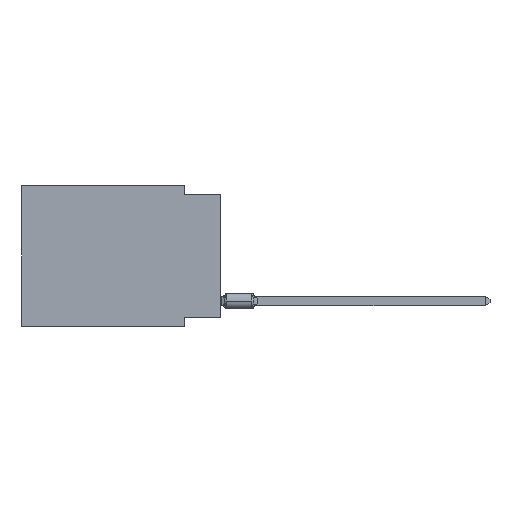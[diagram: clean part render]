
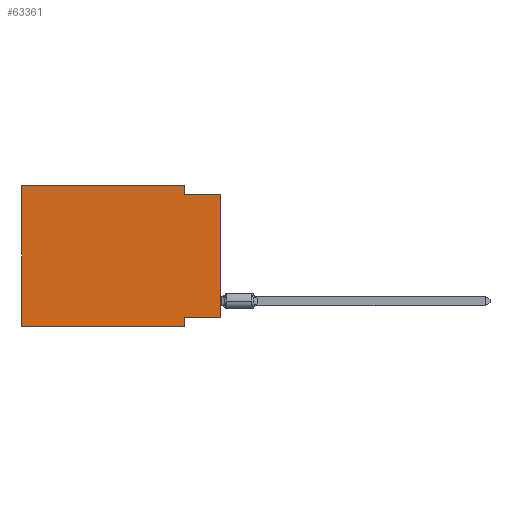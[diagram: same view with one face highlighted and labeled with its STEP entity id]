
A CAD part, left-side view. The second image highlights one B-rep face of the part: STEP entity #63361.
In plain terms, the highlighted planar face has unit normal (-1, 0, 0).
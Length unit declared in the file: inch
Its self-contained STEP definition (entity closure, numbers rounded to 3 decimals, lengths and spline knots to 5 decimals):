
#526 = VECTOR ( 'NONE', #19034, 39.37008 ) ;
#816 = ORIENTED_EDGE ( 'NONE', *, *, #60387, .F. ) ;
#2575 = VERTEX_POINT ( 'NONE', #33905 ) ;
#2750 = VECTOR ( 'NONE', #73653, 39.37008 ) ;
#6491 = CARTESIAN_POINT ( 'NONE',  ( 0., 0.55, 0. ) ) ;
#8063 = EDGE_LOOP ( 'NONE', ( #31172, #16062, #46462, #55585, #9830, #26280, #29709, #816 ) ) ;
#8276 = VERTEX_POINT ( 'NONE', #61489 ) ;
#9830 = ORIENTED_EDGE ( 'NONE', *, *, #71183, .F. ) ;
#11281 = VECTOR ( 'NONE', #72518, 39.37008 ) ;
#12258 = LINE ( 'NONE', #13443, #526 ) ;
#13443 = CARTESIAN_POINT ( 'NONE',  ( 0., 0., 0. ) ) ;
#13620 = LINE ( 'NONE', #6491, #14271 ) ;
#13985 = CARTESIAN_POINT ( 'NONE',  ( 0., 0.1, 0. ) ) ;
#14271 = VECTOR ( 'NONE', #56157, 39.37008 ) ;
#16062 = ORIENTED_EDGE ( 'NONE', *, *, #34835, .F. ) ;
#17043 = VERTEX_POINT ( 'NONE', #25178 ) ;
#17305 = LINE ( 'NONE', #41565, #11281 ) ;
#18023 = LINE ( 'NONE', #37097, #2750 ) ;
#19034 = DIRECTION ( 'NONE',  ( 0., 0., 1. ) ) ;
#19083 = CARTESIAN_POINT ( 'NONE',  ( 0., 0.55, -0.39 ) ) ;
#22002 = LINE ( 'NONE', #28731, #77755 ) ;
#23975 = CARTESIAN_POINT ( 'NONE',  ( 0., 0.1, -0.39 ) ) ;
#25178 = CARTESIAN_POINT ( 'NONE',  ( 0., 0.1, -0.025 ) ) ;
#26280 = ORIENTED_EDGE ( 'NONE', *, *, #65469, .T. ) ;
#28731 = CARTESIAN_POINT ( 'NONE',  ( 0., 0.55, 0. ) ) ;
#29350 = VECTOR ( 'NONE', #68722, 39.37008 ) ;
#29709 = ORIENTED_EDGE ( 'NONE', *, *, #52418, .F. ) ;
#29954 = VERTEX_POINT ( 'NONE', #39991 ) ;
#31172 = ORIENTED_EDGE ( 'NONE', *, *, #39427, .T. ) ;
#33905 = CARTESIAN_POINT ( 'NONE',  ( 0., 0., -0.365 ) ) ;
#34835 = EDGE_CURVE ( 'NONE', #17043, #49606, #18023, .T. ) ;
#35425 = VECTOR ( 'NONE', #44617, 39.37008 ) ;
#37097 = CARTESIAN_POINT ( 'NONE',  ( 0., 0., -0.025 ) ) ;
#39427 = EDGE_CURVE ( 'NONE', #2575, #49606, #12258, .T. ) ;
#39991 = CARTESIAN_POINT ( 'NONE',  ( 0., 0.55, 0. ) ) ;
#40016 = VERTEX_POINT ( 'NONE', #45148 ) ;
#41565 = CARTESIAN_POINT ( 'NONE',  ( 0., 0., -0.365 ) ) ;
#44126 = CARTESIAN_POINT ( 'NONE',  ( 0., 0.1, -0.39 ) ) ;
#44617 = DIRECTION ( 'NONE',  ( 0., 0., -1. ) ) ;
#45148 = CARTESIAN_POINT ( 'NONE',  ( 0., 0.1, -0.365 ) ) ;
#46278 = DIRECTION ( 'NONE',  ( 0., 0., 1. ) ) ;
#46462 = ORIENTED_EDGE ( 'NONE', *, *, #62696, .F. ) ;
#48007 = CARTESIAN_POINT ( 'NONE',  ( 0., 0.55, 0. ) ) ;
#49287 = LINE ( 'NONE', #19083, #29350 ) ;
#49606 = VERTEX_POINT ( 'NONE', #54972 ) ;
#52418 = EDGE_CURVE ( 'NONE', #40016, #58441, #78388, .T. ) ;
#54972 = CARTESIAN_POINT ( 'NONE',  ( 0., 0., -0.025 ) ) ;
#55585 = ORIENTED_EDGE ( 'NONE', *, *, #67926, .F. ) ;
#56157 = DIRECTION ( 'NONE',  ( 0., -1., 0. ) ) ;
#57289 = LINE ( 'NONE', #13985, #35425 ) ;
#58441 = VERTEX_POINT ( 'NONE', #44126 ) ;
#60387 = EDGE_CURVE ( 'NONE', #2575, #40016, #17305, .T. ) ;
#61117 = VERTEX_POINT ( 'NONE', #70690 ) ;
#61489 = CARTESIAN_POINT ( 'NONE',  ( 0., 0.55, -0.39 ) ) ;
#62696 = EDGE_CURVE ( 'NONE', #61117, #17043, #57289, .T. ) ;
#63361 = ADVANCED_FACE ( 'NONE', ( #78163 ), #77776, .F. ) ;
#65469 = EDGE_CURVE ( 'NONE', #8276, #58441, #49287, .T. ) ;
#66254 = DIRECTION ( 'NONE',  ( 0., 0., -1. ) ) ;
#67926 = EDGE_CURVE ( 'NONE', #29954, #61117, #13620, .T. ) ;
#68715 = VECTOR ( 'NONE', #72856, 39.37008 ) ;
#68722 = DIRECTION ( 'NONE',  ( 0., -1., 0. ) ) ;
#70690 = CARTESIAN_POINT ( 'NONE',  ( 0., 0.1, 0. ) ) ;
#71183 = EDGE_CURVE ( 'NONE', #8276, #29954, #22002, .T. ) ;
#72518 = DIRECTION ( 'NONE',  ( 0., 1., 0. ) ) ;
#72856 = DIRECTION ( 'NONE',  ( 0., 0., -1. ) ) ;
#73009 = DIRECTION ( 'NONE',  ( 1., 0., 0. ) ) ;
#73576 = AXIS2_PLACEMENT_3D ( 'NONE', #48007, #73009, #66254 ) ;
#73653 = DIRECTION ( 'NONE',  ( 0., -1., 0. ) ) ;
#77755 = VECTOR ( 'NONE', #46278, 39.37008 ) ;
#77776 = PLANE ( 'NONE',  #73576 ) ;
#78163 = FACE_OUTER_BOUND ( 'NONE', #8063, .T. ) ;
#78388 = LINE ( 'NONE', #23975, #68715 ) ;
